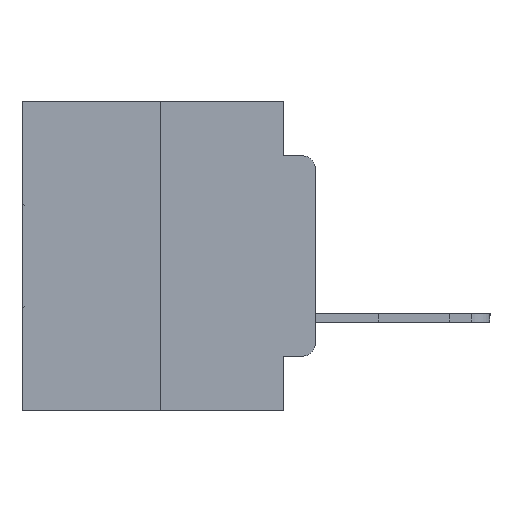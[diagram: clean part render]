
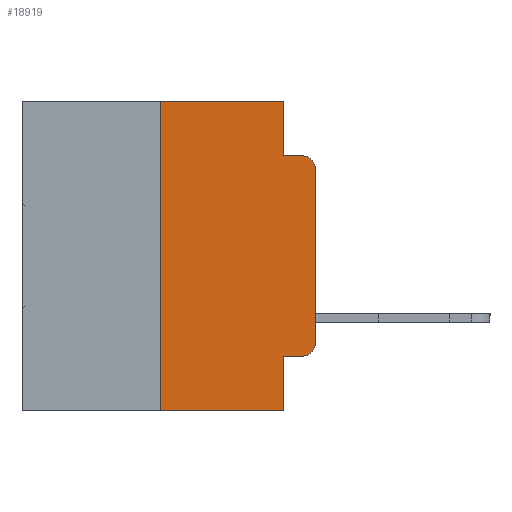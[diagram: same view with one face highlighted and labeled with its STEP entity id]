
A CAD part, left-side view. The second image highlights one B-rep face of the part: STEP entity #18919.
In plain terms, the highlighted planar face has unit normal (-1, 0, 0).
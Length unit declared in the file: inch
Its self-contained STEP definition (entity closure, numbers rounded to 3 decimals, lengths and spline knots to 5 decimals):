
#133 = DIRECTION ( 'NONE',  ( 0., 0., -1. ) ) ;
#172 = VECTOR ( 'NONE', #16532, 39.37008 ) ;
#227 = ORIENTED_EDGE ( 'NONE', *, *, #10884, .F. ) ;
#261 = ORIENTED_EDGE ( 'NONE', *, *, #24505, .F. ) ;
#379 = ORIENTED_EDGE ( 'NONE', *, *, #12571, .F. ) ;
#1806 = VERTEX_POINT ( 'NONE', #21574 ) ;
#2435 = CARTESIAN_POINT ( 'NONE',  ( 0., 0.051, -0.5 ) ) ;
#3529 = CARTESIAN_POINT ( 'NONE',  ( 0., 0.051, -0.0885 ) ) ;
#3631 = DIRECTION ( 'NONE',  ( 0., -1., 0. ) ) ;
#3901 = DIRECTION ( 'NONE',  ( 0., -1., 0. ) ) ;
#3990 = EDGE_CURVE ( 'NONE', #16419, #23910, #11202, .T. ) ;
#4135 = ORIENTED_EDGE ( 'NONE', *, *, #25177, .F. ) ;
#4512 = ORIENTED_EDGE ( 'NONE', *, *, #19613, .T. ) ;
#4574 = LINE ( 'NONE', #25094, #17310 ) ;
#4660 = VERTEX_POINT ( 'NONE', #11350 ) ;
#4986 = ORIENTED_EDGE ( 'NONE', *, *, #3990, .T. ) ;
#5389 = VECTOR ( 'NONE', #3631, 39.37008 ) ;
#5896 = CARTESIAN_POINT ( 'NONE',  ( 0., 0.02, -0.1085 ) ) ;
#6531 = CARTESIAN_POINT ( 'NONE',  ( 0., 0.051, -0.0885 ) ) ;
#6649 = CARTESIAN_POINT ( 'NONE',  ( 0., 0.25, -0.5 ) ) ;
#7757 = LINE ( 'NONE', #29929, #23794 ) ;
#7906 = VERTEX_POINT ( 'NONE', #6649 ) ;
#8105 = DIRECTION ( 'NONE',  ( -1., 0., 0. ) ) ;
#9155 = ORIENTED_EDGE ( 'NONE', *, *, #11932, .T. ) ;
#9264 = EDGE_CURVE ( 'NONE', #16601, #10329, #22399, .T. ) ;
#9652 = CARTESIAN_POINT ( 'NONE',  ( 0., 0.051, -0.4115 ) ) ;
#10329 = VERTEX_POINT ( 'NONE', #2435 ) ;
#10884 = EDGE_CURVE ( 'NONE', #7906, #13724, #19351, .T. ) ;
#11081 = CARTESIAN_POINT ( 'NONE',  ( 0., 0.02, -0.0885 ) ) ;
#11202 = CIRCLE ( 'NONE', #17283, 0.02 ) ;
#11350 = CARTESIAN_POINT ( 'NONE',  ( 0., 0.051, 0. ) ) ;
#11467 = DIRECTION ( 'NONE',  ( 0., 0., -1. ) ) ;
#11671 = LINE ( 'NONE', #3529, #5389 ) ;
#11932 = EDGE_CURVE ( 'NONE', #19227, #16419, #28083, .T. ) ;
#12070 = CARTESIAN_POINT ( 'NONE',  ( 0., 0.051, 0. ) ) ;
#12074 = VERTEX_POINT ( 'NONE', #6531 ) ;
#12158 = ORIENTED_EDGE ( 'NONE', *, *, #30258, .T. ) ;
#12240 = ORIENTED_EDGE ( 'NONE', *, *, #9264, .F. ) ;
#12296 = ORIENTED_EDGE ( 'NONE', *, *, #21181, .T. ) ;
#12427 = CARTESIAN_POINT ( 'NONE',  ( 0., 0.473, 0. ) ) ;
#12571 = EDGE_CURVE ( 'NONE', #4660, #12074, #7757, .T. ) ;
#13650 = LINE ( 'NONE', #24969, #18551 ) ;
#13724 = VERTEX_POINT ( 'NONE', #18236 ) ;
#13745 = DIRECTION ( 'NONE',  ( 0., -1., 0. ) ) ;
#14576 = VECTOR ( 'NONE', #133, 39.37008 ) ;
#14860 = DIRECTION ( 'NONE',  ( 0., 0., -1. ) ) ;
#15908 = CIRCLE ( 'NONE', #16863, 0.02 ) ;
#16419 = VERTEX_POINT ( 'NONE', #27603 ) ;
#16532 = DIRECTION ( 'NONE',  ( 0., 0., 1. ) ) ;
#16601 = VERTEX_POINT ( 'NONE', #9652 ) ;
#16863 = AXIS2_PLACEMENT_3D ( 'NONE', #22482, #8105, #24740 ) ;
#17283 = AXIS2_PLACEMENT_3D ( 'NONE', #5896, #26169, #26577 ) ;
#17310 = VECTOR ( 'NONE', #3901, 39.37008 ) ;
#18236 = CARTESIAN_POINT ( 'NONE',  ( 0., 0.25, 0. ) ) ;
#18551 = VECTOR ( 'NONE', #27177, 39.37008 ) ;
#18919 = ADVANCED_FACE ( 'NONE', ( #26192 ), #28519, .F. ) ;
#19227 = VERTEX_POINT ( 'NONE', #25150 ) ;
#19351 = LINE ( 'NONE', #23647, #172 ) ;
#19613 = EDGE_CURVE ( 'NONE', #1806, #19227, #15908, .T. ) ;
#21181 = EDGE_CURVE ( 'NONE', #16601, #1806, #21579, .T. ) ;
#21574 = CARTESIAN_POINT ( 'NONE',  ( 0., 0.02, -0.4115 ) ) ;
#21579 = LINE ( 'NONE', #25441, #26841 ) ;
#22197 = VECTOR ( 'NONE', #23876, 39.37008 ) ;
#22399 = LINE ( 'NONE', #12070, #14576 ) ;
#22418 = AXIS2_PLACEMENT_3D ( 'NONE', #12427, #28611, #14860 ) ;
#22482 = CARTESIAN_POINT ( 'NONE',  ( 0., 0.02, -0.3915 ) ) ;
#23253 = EDGE_LOOP ( 'NONE', ( #9155, #4986, #4135, #379, #261, #227, #12158, #12240, #12296, #4512 ) ) ;
#23647 = CARTESIAN_POINT ( 'NONE',  ( 0., 0.25, 0. ) ) ;
#23794 = VECTOR ( 'NONE', #11467, 39.37008 ) ;
#23876 = DIRECTION ( 'NONE',  ( 0., 0., 1. ) ) ;
#23910 = VERTEX_POINT ( 'NONE', #11081 ) ;
#24505 = EDGE_CURVE ( 'NONE', #13724, #4660, #13650, .T. ) ;
#24740 = DIRECTION ( 'NONE',  ( 0., 0., -1. ) ) ;
#24969 = CARTESIAN_POINT ( 'NONE',  ( 0., 0.473, 0. ) ) ;
#25094 = CARTESIAN_POINT ( 'NONE',  ( 0., 0.473, -0.5 ) ) ;
#25150 = CARTESIAN_POINT ( 'NONE',  ( 0., 0., -0.3915 ) ) ;
#25177 = EDGE_CURVE ( 'NONE', #12074, #23910, #11671, .T. ) ;
#25420 = CARTESIAN_POINT ( 'NONE',  ( 0., 0., 0. ) ) ;
#25441 = CARTESIAN_POINT ( 'NONE',  ( 0., 0.051, -0.4115 ) ) ;
#26169 = DIRECTION ( 'NONE',  ( -1., 0., 0. ) ) ;
#26192 = FACE_OUTER_BOUND ( 'NONE', #23253, .T. ) ;
#26577 = DIRECTION ( 'NONE',  ( 0., 0., -1. ) ) ;
#26841 = VECTOR ( 'NONE', #13745, 39.37008 ) ;
#27177 = DIRECTION ( 'NONE',  ( 0., -1., 0. ) ) ;
#27603 = CARTESIAN_POINT ( 'NONE',  ( 0., 0., -0.1085 ) ) ;
#28083 = LINE ( 'NONE', #25420, #22197 ) ;
#28519 = PLANE ( 'NONE',  #22418 ) ;
#28611 = DIRECTION ( 'NONE',  ( 1., 0., 0. ) ) ;
#29929 = CARTESIAN_POINT ( 'NONE',  ( 0., 0.051, 0. ) ) ;
#30258 = EDGE_CURVE ( 'NONE', #7906, #10329, #4574, .T. ) ;
